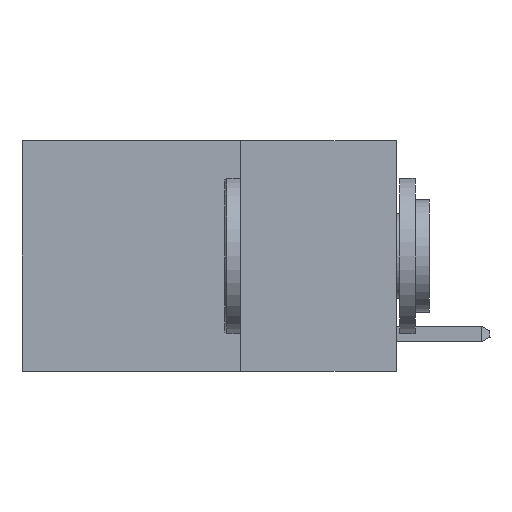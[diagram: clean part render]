
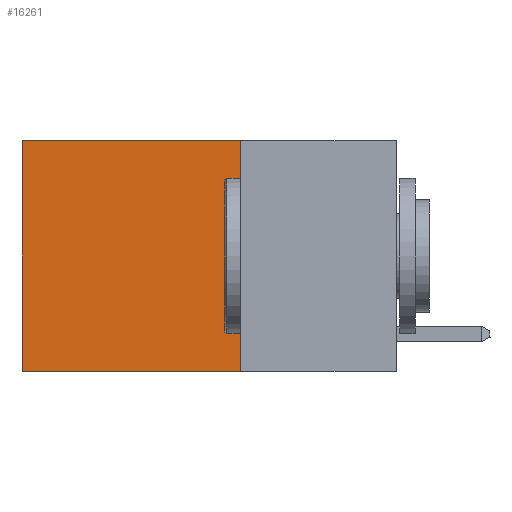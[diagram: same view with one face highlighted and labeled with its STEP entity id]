
A CAD part, left-side view. The second image highlights one B-rep face of the part: STEP entity #16261.
In plain terms, the highlighted planar face has unit normal (-1, 0, 0).
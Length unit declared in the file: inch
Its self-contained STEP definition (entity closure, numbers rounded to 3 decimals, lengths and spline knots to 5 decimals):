
#324 = EDGE_CURVE ( 'NONE', #8594, #24614, #19719, .T. ) ;
#2430 = AXIS2_PLACEMENT_3D ( 'NONE', #17939, #22331, #9535 ) ;
#3575 = DIRECTION ( 'NONE',  ( 0., 1., 0. ) ) ;
#3979 = VECTOR ( 'NONE', #13029, 39.37008 ) ;
#4015 = CARTESIAN_POINT ( 'NONE',  ( 0.2625, 0.25, 0. ) ) ;
#4606 = EDGE_CURVE ( 'NONE', #7453, #19601, #24058, .T. ) ;
#5228 = PLANE ( 'NONE',  #2430 ) ;
#6162 = DIRECTION ( 'NONE',  ( 0., 0., -1. ) ) ;
#6850 = EDGE_LOOP ( 'NONE', ( #9913, #20559, #10327, #10419 ) ) ;
#7453 = VERTEX_POINT ( 'NONE', #15893 ) ;
#7698 = VECTOR ( 'NONE', #24170, 39.37008 ) ;
#8594 = VERTEX_POINT ( 'NONE', #9105 ) ;
#9105 = CARTESIAN_POINT ( 'NONE',  ( 0.2625, 0.25, -0.37 ) ) ;
#9535 = DIRECTION ( 'NONE',  ( 0., 0., -1. ) ) ;
#9571 = EDGE_CURVE ( 'NONE', #7453, #8594, #22078, .T. ) ;
#9598 = CARTESIAN_POINT ( 'NONE',  ( 0.2625, 0.6, 0. ) ) ;
#9913 = ORIENTED_EDGE ( 'NONE', *, *, #23713, .T. ) ;
#10327 = ORIENTED_EDGE ( 'NONE', *, *, #9571, .F. ) ;
#10419 = ORIENTED_EDGE ( 'NONE', *, *, #4606, .T. ) ;
#12531 = FACE_OUTER_BOUND ( 'NONE', #6850, .T. ) ;
#12700 = VECTOR ( 'NONE', #3575, 39.37008 ) ;
#13029 = DIRECTION ( 'NONE',  ( 0., 0., -1. ) ) ;
#15093 = CARTESIAN_POINT ( 'NONE',  ( 0.2625, 0.6, 0. ) ) ;
#15893 = CARTESIAN_POINT ( 'NONE',  ( 0.2625, 0.25, 0. ) ) ;
#15965 = CARTESIAN_POINT ( 'NONE',  ( 0.2625, 0.6, -0.37 ) ) ;
#16261 = ADVANCED_FACE ( 'NONE', ( #12531 ), #5228, .F. ) ;
#16371 = CARTESIAN_POINT ( 'NONE',  ( 0.2625, 0.25, 0. ) ) ;
#17825 = CARTESIAN_POINT ( 'NONE',  ( 0.2625, 0.25, -0.37 ) ) ;
#17939 = CARTESIAN_POINT ( 'NONE',  ( 0.2625, 0.25, 0. ) ) ;
#19601 = VERTEX_POINT ( 'NONE', #9598 ) ;
#19719 = LINE ( 'NONE', #17825, #7698 ) ;
#20559 = ORIENTED_EDGE ( 'NONE', *, *, #324, .F. ) ;
#21037 = LINE ( 'NONE', #15093, #3979 ) ;
#21415 = VECTOR ( 'NONE', #6162, 39.37008 ) ;
#22078 = LINE ( 'NONE', #4015, #21415 ) ;
#22331 = DIRECTION ( 'NONE',  ( 1., 0., 0. ) ) ;
#23713 = EDGE_CURVE ( 'NONE', #19601, #24614, #21037, .T. ) ;
#24058 = LINE ( 'NONE', #16371, #12700 ) ;
#24170 = DIRECTION ( 'NONE',  ( 0., 1., 0. ) ) ;
#24614 = VERTEX_POINT ( 'NONE', #15965 ) ;
